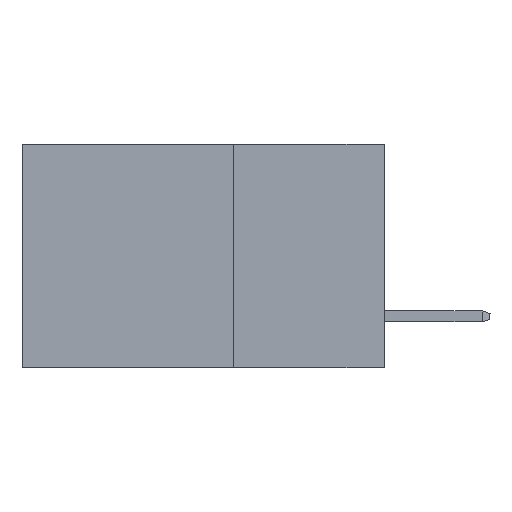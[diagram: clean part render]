
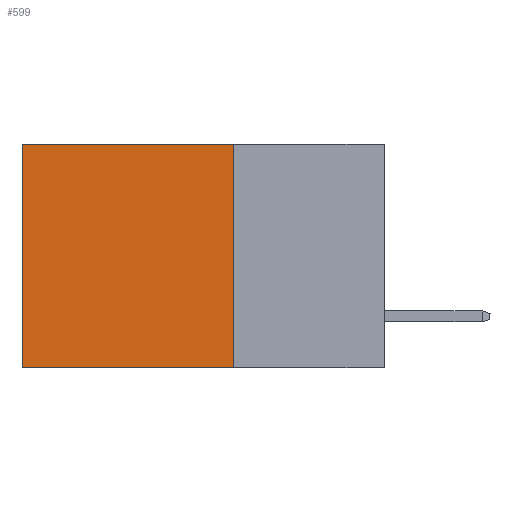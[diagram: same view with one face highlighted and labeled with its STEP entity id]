
A CAD part, left-side view. The second image highlights one B-rep face of the part: STEP entity #599.
In plain terms, the highlighted planar face has unit normal (-1, 0, 0).
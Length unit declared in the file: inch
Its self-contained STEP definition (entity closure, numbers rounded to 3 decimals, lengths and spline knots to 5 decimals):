
#28 = EDGE_CURVE ( 'NONE', #11782, #6315, #5509, .T. ) ;
#599 = ADVANCED_FACE ( 'NONE', ( #3650 ), #1081, .F. ) ;
#871 = DIRECTION ( 'NONE',  ( 1., 0., 0. ) ) ;
#963 = ORIENTED_EDGE ( 'NONE', *, *, #9540, .T. ) ;
#1081 = PLANE ( 'NONE',  #17293 ) ;
#1744 = VECTOR ( 'NONE', #11107, 39.37008 ) ;
#3138 = LINE ( 'NONE', #3334, #13799 ) ;
#3334 = CARTESIAN_POINT ( 'NONE',  ( 0.2615, 0.25, 0. ) ) ;
#3590 = CARTESIAN_POINT ( 'NONE',  ( 0.2615, 0.6, -0.37 ) ) ;
#3612 = ORIENTED_EDGE ( 'NONE', *, *, #13422, .T. ) ;
#3650 = FACE_OUTER_BOUND ( 'NONE', #11152, .T. ) ;
#4043 = CARTESIAN_POINT ( 'NONE',  ( 0.2615, 0.25, -0.37 ) ) ;
#4569 = CARTESIAN_POINT ( 'NONE',  ( 0.2615, 0.25, -0.37 ) ) ;
#5086 = CARTESIAN_POINT ( 'NONE',  ( 0.2615, 0.25, -0.37 ) ) ;
#5509 = LINE ( 'NONE', #16996, #8515 ) ;
#6315 = VERTEX_POINT ( 'NONE', #9834 ) ;
#6393 = VECTOR ( 'NONE', #6576, 39.37008 ) ;
#6576 = DIRECTION ( 'NONE',  ( 0., 0., -1. ) ) ;
#7684 = DIRECTION ( 'NONE',  ( 0., 1., 0. ) ) ;
#7742 = ORIENTED_EDGE ( 'NONE', *, *, #28, .F. ) ;
#8185 = DIRECTION ( 'NONE',  ( 0., 0., -1. ) ) ;
#8515 = VECTOR ( 'NONE', #18704, 39.37008 ) ;
#9517 = ORIENTED_EDGE ( 'NONE', *, *, #14866, .F. ) ;
#9540 = EDGE_CURVE ( 'NONE', #16359, #10948, #3138, .T. ) ;
#9659 = CARTESIAN_POINT ( 'NONE',  ( 0.2615, 0.6, 0. ) ) ;
#9800 = LINE ( 'NONE', #3590, #6393 ) ;
#9834 = CARTESIAN_POINT ( 'NONE',  ( 0.2615, 0.6, -0.37 ) ) ;
#10948 = VERTEX_POINT ( 'NONE', #9659 ) ;
#11107 = DIRECTION ( 'NONE',  ( 0., 0., -1. ) ) ;
#11152 = EDGE_LOOP ( 'NONE', ( #3612, #7742, #9517, #963 ) ) ;
#11782 = VERTEX_POINT ( 'NONE', #4569 ) ;
#13422 = EDGE_CURVE ( 'NONE', #10948, #6315, #9800, .T. ) ;
#13799 = VECTOR ( 'NONE', #7684, 39.37008 ) ;
#14866 = EDGE_CURVE ( 'NONE', #16359, #11782, #18578, .T. ) ;
#15275 = CARTESIAN_POINT ( 'NONE',  ( 0.2615, 0.25, 0. ) ) ;
#16359 = VERTEX_POINT ( 'NONE', #15275 ) ;
#16996 = CARTESIAN_POINT ( 'NONE',  ( 0.2615, 0.25, -0.37 ) ) ;
#17293 = AXIS2_PLACEMENT_3D ( 'NONE', #4043, #871, #8185 ) ;
#18578 = LINE ( 'NONE', #5086, #1744 ) ;
#18704 = DIRECTION ( 'NONE',  ( 0., 1., 0. ) ) ;
